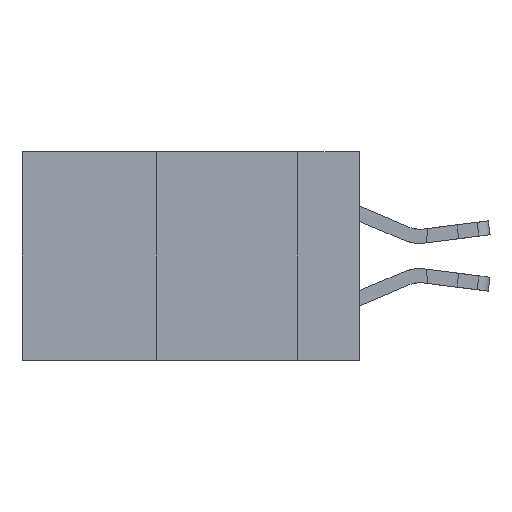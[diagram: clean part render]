
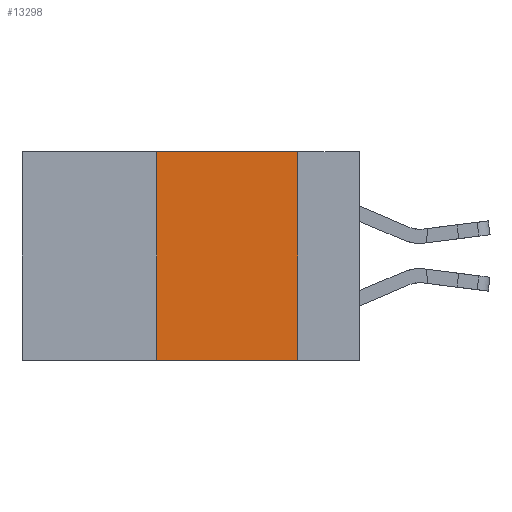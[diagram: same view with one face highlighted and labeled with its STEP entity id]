
A CAD part, left-side view. The second image highlights one B-rep face of the part: STEP entity #13298.
In plain terms, the highlighted planar face has unit normal (-1, 0, 0).
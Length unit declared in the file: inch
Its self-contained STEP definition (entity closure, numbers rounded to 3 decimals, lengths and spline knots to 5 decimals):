
#244 = DIRECTION ( 'NONE',  ( 0., 0., -1. ) ) ;
#457 = VECTOR ( 'NONE', #19240, 39.37008 ) ;
#506 = EDGE_CURVE ( 'NONE', #14177, #4363, #7476, .T. ) ;
#523 = CARTESIAN_POINT ( 'NONE',  ( 0., 0.6, 0. ) ) ;
#1925 = EDGE_CURVE ( 'NONE', #14177, #9886, #11424, .T. ) ;
#2595 = VECTOR ( 'NONE', #18856, 39.37008 ) ;
#3907 = PLANE ( 'NONE',  #4165 ) ;
#4165 = AXIS2_PLACEMENT_3D ( 'NONE', #11188, #11271, #244 ) ;
#4363 = VERTEX_POINT ( 'NONE', #22900 ) ;
#5484 = VECTOR ( 'NONE', #20640, 39.37008 ) ;
#7476 = LINE ( 'NONE', #13396, #2595 ) ;
#8672 = ORIENTED_EDGE ( 'NONE', *, *, #506, .T. ) ;
#8852 = EDGE_CURVE ( 'NONE', #9886, #19060, #10347, .T. ) ;
#8974 = FACE_OUTER_BOUND ( 'NONE', #16275, .T. ) ;
#9886 = VERTEX_POINT ( 'NONE', #21466 ) ;
#10347 = LINE ( 'NONE', #523, #5484 ) ;
#11188 = CARTESIAN_POINT ( 'NONE',  ( 0., 0.6, 0. ) ) ;
#11271 = DIRECTION ( 'NONE',  ( 1., 0., 0. ) ) ;
#11424 = LINE ( 'NONE', #15465, #16263 ) ;
#11811 = DIRECTION ( 'NONE',  ( 0., 0., 1. ) ) ;
#13223 = CARTESIAN_POINT ( 'NONE',  ( 0., 0.11, 0. ) ) ;
#13298 = ADVANCED_FACE ( 'NONE', ( #8974 ), #3907, .F. ) ;
#13396 = CARTESIAN_POINT ( 'NONE',  ( 0., 0.6, -0.37 ) ) ;
#14177 = VERTEX_POINT ( 'NONE', #19089 ) ;
#15465 = CARTESIAN_POINT ( 'NONE',  ( 0., 0.36, 0. ) ) ;
#16263 = VECTOR ( 'NONE', #11811, 39.37008 ) ;
#16275 = EDGE_LOOP ( 'NONE', ( #21152, #22249, #19730, #8672 ) ) ;
#17272 = EDGE_CURVE ( 'NONE', #19060, #4363, #19335, .T. ) ;
#18856 = DIRECTION ( 'NONE',  ( 0., -1., 0. ) ) ;
#19060 = VERTEX_POINT ( 'NONE', #13223 ) ;
#19089 = CARTESIAN_POINT ( 'NONE',  ( 0., 0.36, -0.37 ) ) ;
#19240 = DIRECTION ( 'NONE',  ( 0., 0., -1. ) ) ;
#19335 = LINE ( 'NONE', #22821, #457 ) ;
#19730 = ORIENTED_EDGE ( 'NONE', *, *, #1925, .F. ) ;
#20640 = DIRECTION ( 'NONE',  ( 0., -1., 0. ) ) ;
#21152 = ORIENTED_EDGE ( 'NONE', *, *, #17272, .F. ) ;
#21466 = CARTESIAN_POINT ( 'NONE',  ( 0., 0.36, 0. ) ) ;
#22249 = ORIENTED_EDGE ( 'NONE', *, *, #8852, .F. ) ;
#22821 = CARTESIAN_POINT ( 'NONE',  ( 0., 0.11, 0. ) ) ;
#22900 = CARTESIAN_POINT ( 'NONE',  ( 0., 0.11, -0.37 ) ) ;
